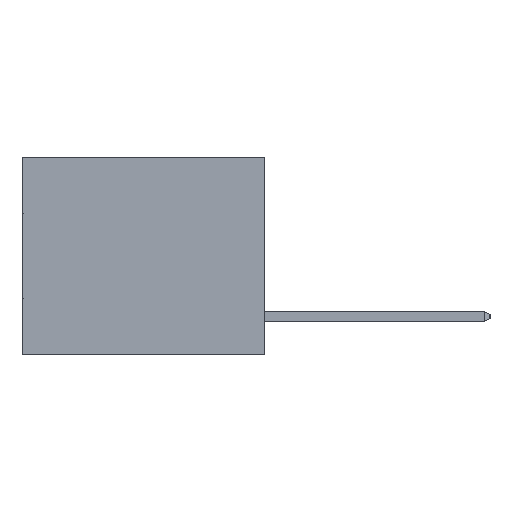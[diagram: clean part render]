
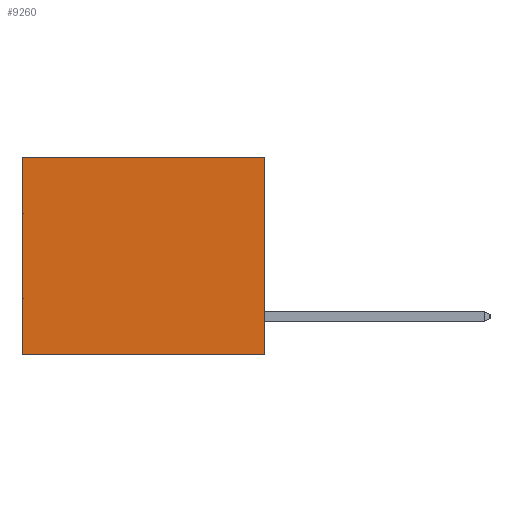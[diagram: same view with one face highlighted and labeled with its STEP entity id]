
A CAD part, left-side view. The second image highlights one B-rep face of the part: STEP entity #9260.
In plain terms, the highlighted planar face has unit normal (-1, 0, 0).
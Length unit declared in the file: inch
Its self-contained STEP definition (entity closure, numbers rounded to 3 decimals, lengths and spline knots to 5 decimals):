
#912 = ORIENTED_EDGE ( 'NONE', *, *, #32201, .F. ) ;
#1046 = LINE ( 'NONE', #4173, #2262 ) ;
#2180 = DIRECTION ( 'NONE',  ( 0., 0., -1. ) ) ;
#2262 = VECTOR ( 'NONE', #30491, 39.37008 ) ;
#2376 = EDGE_CURVE ( 'NONE', #9501, #7463, #12100, .T. ) ;
#4173 = CARTESIAN_POINT ( 'NONE',  ( 0.3165, 0., -0.49 ) ) ;
#4484 = VECTOR ( 'NONE', #17600, 39.37008 ) ;
#4595 = CARTESIAN_POINT ( 'NONE',  ( 0.3165, 0.6, -0.49 ) ) ;
#5774 = CARTESIAN_POINT ( 'NONE',  ( 0.3165, 0.6, -0.49 ) ) ;
#5893 = ORIENTED_EDGE ( 'NONE', *, *, #27625, .F. ) ;
#6847 = LINE ( 'NONE', #10316, #22693 ) ;
#7463 = VERTEX_POINT ( 'NONE', #5774 ) ;
#7862 = CARTESIAN_POINT ( 'NONE',  ( 0.3165, 0., 0. ) ) ;
#9260 = ADVANCED_FACE ( 'NONE', ( #31233 ), #14127, .F. ) ;
#9501 = VERTEX_POINT ( 'NONE', #29326 ) ;
#10316 = CARTESIAN_POINT ( 'NONE',  ( 0.3165, 0., -0.49 ) ) ;
#11731 = DIRECTION ( 'NONE',  ( 0., 0., -1. ) ) ;
#12100 = LINE ( 'NONE', #4595, #16582 ) ;
#12483 = CARTESIAN_POINT ( 'NONE',  ( 0.3165, 0., 0. ) ) ;
#13382 = EDGE_LOOP ( 'NONE', ( #22703, #5893, #912, #27700 ) ) ;
#14127 = PLANE ( 'NONE',  #31970 ) ;
#16550 = EDGE_CURVE ( 'NONE', #29490, #9501, #33271, .T. ) ;
#16582 = VECTOR ( 'NONE', #2180, 39.37008 ) ;
#17600 = DIRECTION ( 'NONE',  ( 0., 1., 0. ) ) ;
#19561 = CARTESIAN_POINT ( 'NONE',  ( 0.3165, 0., -0.49 ) ) ;
#21252 = VERTEX_POINT ( 'NONE', #27604 ) ;
#22693 = VECTOR ( 'NONE', #24057, 39.37008 ) ;
#22703 = ORIENTED_EDGE ( 'NONE', *, *, #2376, .T. ) ;
#24057 = DIRECTION ( 'NONE',  ( 0., 0., -1. ) ) ;
#27604 = CARTESIAN_POINT ( 'NONE',  ( 0.3165, 0., -0.49 ) ) ;
#27625 = EDGE_CURVE ( 'NONE', #21252, #7463, #1046, .T. ) ;
#27700 = ORIENTED_EDGE ( 'NONE', *, *, #16550, .T. ) ;
#29326 = CARTESIAN_POINT ( 'NONE',  ( 0.3165, 0.6, 0. ) ) ;
#29490 = VERTEX_POINT ( 'NONE', #7862 ) ;
#29606 = DIRECTION ( 'NONE',  ( 1., 0., 0. ) ) ;
#30491 = DIRECTION ( 'NONE',  ( 0., 1., 0. ) ) ;
#31233 = FACE_OUTER_BOUND ( 'NONE', #13382, .T. ) ;
#31970 = AXIS2_PLACEMENT_3D ( 'NONE', #19561, #29606, #11731 ) ;
#32201 = EDGE_CURVE ( 'NONE', #29490, #21252, #6847, .T. ) ;
#33271 = LINE ( 'NONE', #12483, #4484 ) ;
